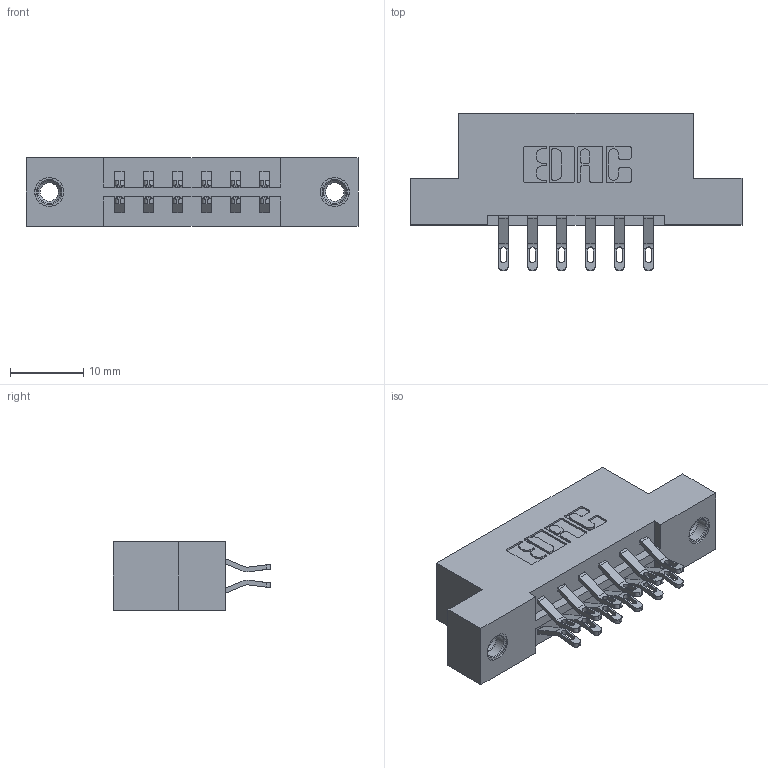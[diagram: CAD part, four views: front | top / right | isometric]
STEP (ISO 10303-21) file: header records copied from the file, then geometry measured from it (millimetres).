
FILE_DESCRIPTION (( 'STEP AP203' ), '1' );
FILE_NAME ('833-012-555-207.STEP', '2020-05-30T22:34:12', ( '' ), ( '' ), 'SwSTEP 2.0', 'SolidWorks 2020', '' );
FILE_SCHEMA (( 'CONFIG_CONTROL_DESIGN' ));
Length unit declared in the file: inch
Products named in the file (4): 833-012-555-207; 833 Part_Flush - .156 Dia - TI; 345-292-001_555 Tail; 345-250-001_345-250-005-103
Assembly tree (15 placements, depth 2):
  833-012-555-207
    833 Part_Flush - .156 Dia - TI
    345-292-001_555 Tail  x12
    345-250-001_345-250-005-103  x2
Bounding box: 45.31 x 21.47 x 9.4 mm (x, y, z)
Volume: 4310.9 mm3; surface area: 4874 mm2
Topology: 15 solids, 15 shells, 870 faces, 2643 edges, 1754 vertices
Faces by surface type: plane 510, cylinder 344, cone 12, torus 4
Entity records: 10028 total; most frequent: CARTESIAN_POINT 1723, ORIENTED_EDGE 1622, DIRECTION 1537, EDGE_CURVE 811, LINE 643, VECTOR 643, VERTEX_POINT 536, AXIS2_PLACEMENT_3D 447
